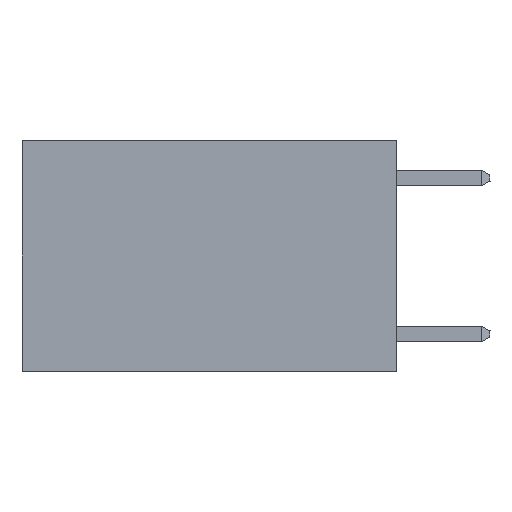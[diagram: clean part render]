
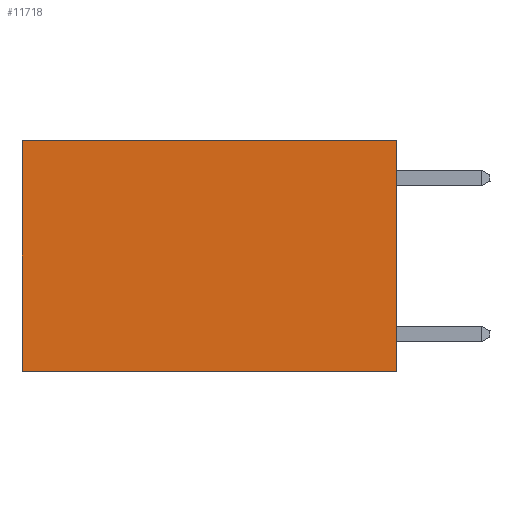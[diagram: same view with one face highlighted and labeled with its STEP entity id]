
A CAD part, left-side view. The second image highlights one B-rep face of the part: STEP entity #11718.
In plain terms, the highlighted planar face has unit normal (-1, 0, 0).
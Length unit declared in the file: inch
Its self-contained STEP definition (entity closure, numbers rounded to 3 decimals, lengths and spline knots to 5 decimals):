
#706 = CARTESIAN_POINT ( 'NONE',  ( 0.2625, 0.6, 0. ) ) ;
#1075 = LINE ( 'NONE', #8613, #11835 ) ;
#1217 = CARTESIAN_POINT ( 'NONE',  ( 0.2625, 0., -0.37 ) ) ;
#1307 = EDGE_CURVE ( 'NONE', #9813, #6850, #7190, .T. ) ;
#1579 = CARTESIAN_POINT ( 'NONE',  ( 0.2625, 0., 0. ) ) ;
#2583 = VECTOR ( 'NONE', #9816, 39.37008 ) ;
#2682 = DIRECTION ( 'NONE',  ( 1., 0., 0. ) ) ;
#3109 = VECTOR ( 'NONE', #7725, 39.37008 ) ;
#3217 = EDGE_CURVE ( 'NONE', #6850, #10998, #11752, .T. ) ;
#4217 = CARTESIAN_POINT ( 'NONE',  ( 0.2625, 0., 0. ) ) ;
#4905 = EDGE_CURVE ( 'NONE', #10400, #10998, #1075, .T. ) ;
#4932 = AXIS2_PLACEMENT_3D ( 'NONE', #5408, #2682, #6367 ) ;
#5408 = CARTESIAN_POINT ( 'NONE',  ( 0.2625, 0., 0. ) ) ;
#5741 = CARTESIAN_POINT ( 'NONE',  ( 0.2625, 0., 0. ) ) ;
#6095 = CARTESIAN_POINT ( 'NONE',  ( 0.2625, 0.6, -0.37 ) ) ;
#6225 = ORIENTED_EDGE ( 'NONE', *, *, #1307, .F. ) ;
#6302 = EDGE_LOOP ( 'NONE', ( #11222, #8064, #6225, #11349 ) ) ;
#6367 = DIRECTION ( 'NONE',  ( 0., 0., -1. ) ) ;
#6850 = VERTEX_POINT ( 'NONE', #11371 ) ;
#7190 = LINE ( 'NONE', #4217, #2583 ) ;
#7725 = DIRECTION ( 'NONE',  ( 0., 1., 0. ) ) ;
#8064 = ORIENTED_EDGE ( 'NONE', *, *, #3217, .F. ) ;
#8131 = EDGE_CURVE ( 'NONE', #9813, #10400, #11216, .T. ) ;
#8613 = CARTESIAN_POINT ( 'NONE',  ( 0.2625, 0.6, 0. ) ) ;
#8675 = DIRECTION ( 'NONE',  ( 0., 0., -1. ) ) ;
#8848 = VECTOR ( 'NONE', #9792, 39.37008 ) ;
#9792 = DIRECTION ( 'NONE',  ( 0., 1., 0. ) ) ;
#9813 = VERTEX_POINT ( 'NONE', #1579 ) ;
#9816 = DIRECTION ( 'NONE',  ( 0., 0., -1. ) ) ;
#10400 = VERTEX_POINT ( 'NONE', #706 ) ;
#10998 = VERTEX_POINT ( 'NONE', #6095 ) ;
#11138 = PLANE ( 'NONE',  #4932 ) ;
#11216 = LINE ( 'NONE', #5741, #3109 ) ;
#11222 = ORIENTED_EDGE ( 'NONE', *, *, #4905, .T. ) ;
#11349 = ORIENTED_EDGE ( 'NONE', *, *, #8131, .T. ) ;
#11371 = CARTESIAN_POINT ( 'NONE',  ( 0.2625, 0., -0.37 ) ) ;
#11718 = ADVANCED_FACE ( 'NONE', ( #12123 ), #11138, .F. ) ;
#11752 = LINE ( 'NONE', #1217, #8848 ) ;
#11835 = VECTOR ( 'NONE', #8675, 39.37008 ) ;
#12123 = FACE_OUTER_BOUND ( 'NONE', #6302, .T. ) ;
